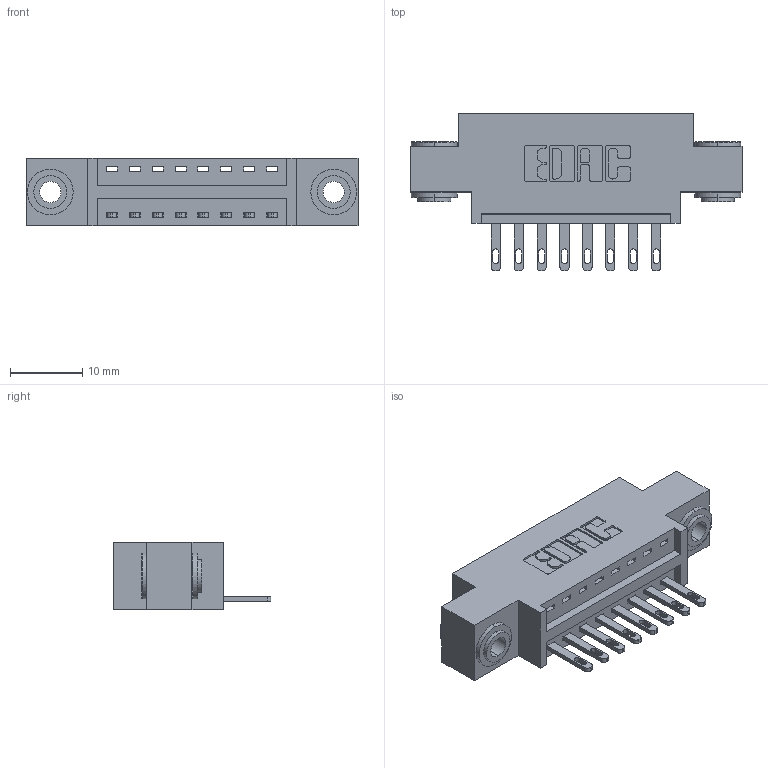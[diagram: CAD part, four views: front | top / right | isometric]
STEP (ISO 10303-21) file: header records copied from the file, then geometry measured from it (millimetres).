
FILE_DESCRIPTION (( 'STEP AP203' ), '1' );
FILE_NAME ('346-008-500-603.STEP', '2018-08-17T04:24:02', ( '' ), ( '' ), 'SwSTEP 2.0', 'SolidWorks 2016', '' );
FILE_SCHEMA (( 'CONFIG_CONTROL_DESIGN' ));
Length unit declared in the file: inch
Products named in the file (4): 345-250-002_345-250-002-102; 346-008-500-603; 346 Part_0.170 Offset - 0.156 Dia-TH; 345-292-001_345-293-100
Assembly tree (11 placements, depth 2):
  346-008-500-603
    346 Part_0.170 Offset - 0.156 Dia-TH
    345-292-001_345-293-100  x8
    345-250-002_345-250-002-102  x2
Bounding box: 45.97 x 21.84 x 9.4 mm (x, y, z)
Volume: 4036.2 mm3; surface area: 5076 mm2
Topology: 11 solids, 11 shells, 596 faces, 1761 edges, 1170 vertices
Faces by surface type: plane 362, cylinder 226, cone 8
Entity records: 10254 total; most frequent: CARTESIAN_POINT 1747, ORIENTED_EDGE 1682, DIRECTION 1615, EDGE_CURVE 841, LINE 649, VECTOR 649, VERTEX_POINT 558, AXIS2_PLACEMENT_3D 483
